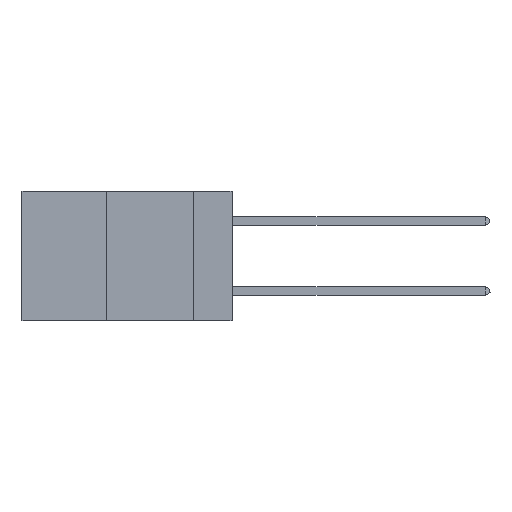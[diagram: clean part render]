
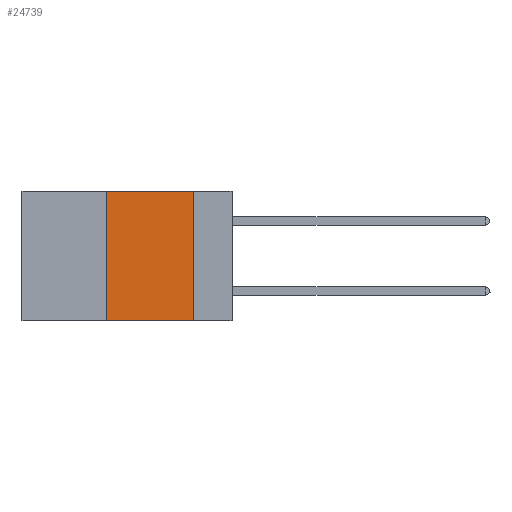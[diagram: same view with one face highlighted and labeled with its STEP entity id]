
A CAD part, left-side view. The second image highlights one B-rep face of the part: STEP entity #24739.
In plain terms, the highlighted planar face has unit normal (-1, 0, 0).
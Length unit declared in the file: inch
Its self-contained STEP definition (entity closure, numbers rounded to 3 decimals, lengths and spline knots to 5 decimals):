
#657 = VERTEX_POINT ( 'NONE', #13807 ) ;
#981 = EDGE_CURVE ( 'NONE', #5961, #657, #3912, .T. ) ;
#1176 = ORIENTED_EDGE ( 'NONE', *, *, #3132, .F. ) ;
#1762 = CARTESIAN_POINT ( 'NONE',  ( 0., 0.36, -0.37 ) ) ;
#1800 = DIRECTION ( 'NONE',  ( 0., -1., 0. ) ) ;
#2420 = VECTOR ( 'NONE', #15871, 39.37008 ) ;
#2810 = VERTEX_POINT ( 'NONE', #4063 ) ;
#3132 = EDGE_CURVE ( 'NONE', #14079, #657, #7143, .T. ) ;
#3341 = PLANE ( 'NONE',  #23902 ) ;
#3912 = LINE ( 'NONE', #14735, #6935 ) ;
#4063 = CARTESIAN_POINT ( 'NONE',  ( 0., 0.36, 0. ) ) ;
#4119 = DIRECTION ( 'NONE',  ( 0., -1., 0. ) ) ;
#4555 = CARTESIAN_POINT ( 'NONE',  ( 0., 0.11, 0. ) ) ;
#4807 = VECTOR ( 'NONE', #23049, 39.37008 ) ;
#5227 = ORIENTED_EDGE ( 'NONE', *, *, #27643, .F. ) ;
#5961 = VERTEX_POINT ( 'NONE', #1762 ) ;
#6935 = VECTOR ( 'NONE', #4119, 39.37008 ) ;
#7143 = LINE ( 'NONE', #26787, #2420 ) ;
#8306 = VECTOR ( 'NONE', #1800, 39.37008 ) ;
#11783 = DIRECTION ( 'NONE',  ( 1., 0., 0. ) ) ;
#12049 = CARTESIAN_POINT ( 'NONE',  ( 0., 0.36, 0. ) ) ;
#12719 = EDGE_CURVE ( 'NONE', #2810, #14079, #24772, .T. ) ;
#13807 = CARTESIAN_POINT ( 'NONE',  ( 0., 0.11, -0.37 ) ) ;
#14079 = VERTEX_POINT ( 'NONE', #4555 ) ;
#14735 = CARTESIAN_POINT ( 'NONE',  ( 0., 0.6, -0.37 ) ) ;
#14957 = CARTESIAN_POINT ( 'NONE',  ( 0., 0.6, 0. ) ) ;
#15871 = DIRECTION ( 'NONE',  ( 0., 0., -1. ) ) ;
#16375 = CARTESIAN_POINT ( 'NONE',  ( 0., 0.6, 0. ) ) ;
#17222 = LINE ( 'NONE', #12049, #4807 ) ;
#19288 = EDGE_LOOP ( 'NONE', ( #1176, #20760, #5227, #21040 ) ) ;
#20760 = ORIENTED_EDGE ( 'NONE', *, *, #12719, .F. ) ;
#21040 = ORIENTED_EDGE ( 'NONE', *, *, #981, .T. ) ;
#23049 = DIRECTION ( 'NONE',  ( 0., 0., 1. ) ) ;
#23902 = AXIS2_PLACEMENT_3D ( 'NONE', #16375, #11783, #24672 ) ;
#24672 = DIRECTION ( 'NONE',  ( 0., 0., -1. ) ) ;
#24739 = ADVANCED_FACE ( 'NONE', ( #27644 ), #3341, .F. ) ;
#24772 = LINE ( 'NONE', #14957, #8306 ) ;
#26787 = CARTESIAN_POINT ( 'NONE',  ( 0., 0.11, 0. ) ) ;
#27643 = EDGE_CURVE ( 'NONE', #5961, #2810, #17222, .T. ) ;
#27644 = FACE_OUTER_BOUND ( 'NONE', #19288, .T. ) ;
